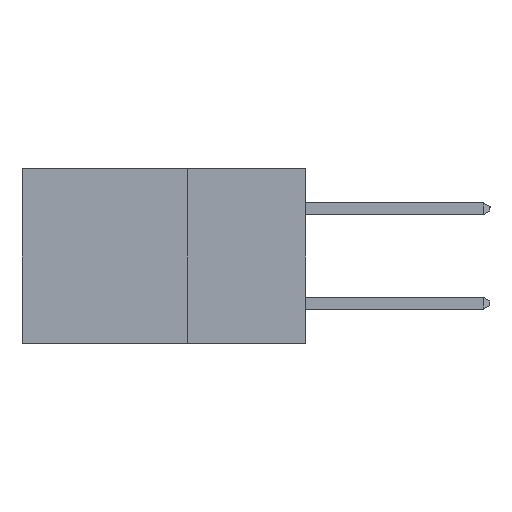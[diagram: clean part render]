
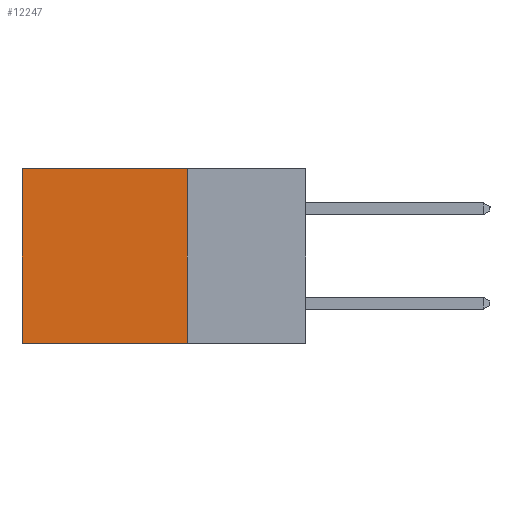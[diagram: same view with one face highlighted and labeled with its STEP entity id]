
A CAD part, left-side view. The second image highlights one B-rep face of the part: STEP entity #12247.
In plain terms, the highlighted planar face has unit normal (-1, 0, 0).
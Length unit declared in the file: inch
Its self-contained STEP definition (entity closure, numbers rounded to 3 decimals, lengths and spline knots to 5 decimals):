
#1269 = DIRECTION ( 'NONE',  ( 1., 0., 0. ) ) ;
#1319 = LINE ( 'NONE', #7645, #9529 ) ;
#2458 = CARTESIAN_POINT ( 'NONE',  ( 0.2615, 0.25, 0. ) ) ;
#2555 = AXIS2_PLACEMENT_3D ( 'NONE', #15437, #1269, #20169 ) ;
#2653 = DIRECTION ( 'NONE',  ( 0., 1., 0. ) ) ;
#2869 = VERTEX_POINT ( 'NONE', #17531 ) ;
#3070 = CARTESIAN_POINT ( 'NONE',  ( 0.2615, 0.25, -0.37 ) ) ;
#3298 = ORIENTED_EDGE ( 'NONE', *, *, #4735, .F. ) ;
#3347 = CARTESIAN_POINT ( 'NONE',  ( 0.2615, 0.6, -0.37 ) ) ;
#3699 = VECTOR ( 'NONE', #5896, 39.37008 ) ;
#3778 = ORIENTED_EDGE ( 'NONE', *, *, #15554, .T. ) ;
#3806 = VERTEX_POINT ( 'NONE', #6261 ) ;
#3885 = EDGE_LOOP ( 'NONE', ( #3778, #19081, #3298, #16206 ) ) ;
#4219 = VECTOR ( 'NONE', #7930, 39.37008 ) ;
#4735 = EDGE_CURVE ( 'NONE', #3806, #17805, #12768, .T. ) ;
#4915 = LINE ( 'NONE', #3347, #7464 ) ;
#5024 = DIRECTION ( 'NONE',  ( 0., 0., -1. ) ) ;
#5896 = DIRECTION ( 'NONE',  ( 0., 1., 0. ) ) ;
#6261 = CARTESIAN_POINT ( 'NONE',  ( 0.2615, 0.25, 0. ) ) ;
#7464 = VECTOR ( 'NONE', #5024, 39.37008 ) ;
#7645 = CARTESIAN_POINT ( 'NONE',  ( 0.2615, 0.25, -0.37 ) ) ;
#7930 = DIRECTION ( 'NONE',  ( 0., 0., -1. ) ) ;
#8716 = EDGE_CURVE ( 'NONE', #17805, #2869, #1319, .T. ) ;
#9115 = PLANE ( 'NONE',  #2555 ) ;
#9529 = VECTOR ( 'NONE', #2653, 39.37008 ) ;
#10677 = FACE_OUTER_BOUND ( 'NONE', #3885, .T. ) ;
#12247 = ADVANCED_FACE ( 'NONE', ( #10677 ), #9115, .F. ) ;
#12406 = CARTESIAN_POINT ( 'NONE',  ( 0.2615, 0.6, 0. ) ) ;
#12595 = VERTEX_POINT ( 'NONE', #12406 ) ;
#12768 = LINE ( 'NONE', #3070, #4219 ) ;
#15437 = CARTESIAN_POINT ( 'NONE',  ( 0.2615, 0.25, -0.37 ) ) ;
#15527 = CARTESIAN_POINT ( 'NONE',  ( 0.2615, 0.25, -0.37 ) ) ;
#15554 = EDGE_CURVE ( 'NONE', #12595, #2869, #4915, .T. ) ;
#16206 = ORIENTED_EDGE ( 'NONE', *, *, #16824, .T. ) ;
#16824 = EDGE_CURVE ( 'NONE', #3806, #12595, #19614, .T. ) ;
#17531 = CARTESIAN_POINT ( 'NONE',  ( 0.2615, 0.6, -0.37 ) ) ;
#17805 = VERTEX_POINT ( 'NONE', #15527 ) ;
#19081 = ORIENTED_EDGE ( 'NONE', *, *, #8716, .F. ) ;
#19614 = LINE ( 'NONE', #2458, #3699 ) ;
#20169 = DIRECTION ( 'NONE',  ( 0., 0., -1. ) ) ;
